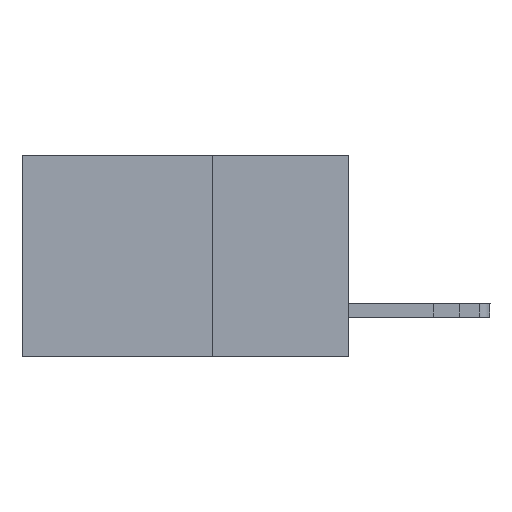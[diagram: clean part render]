
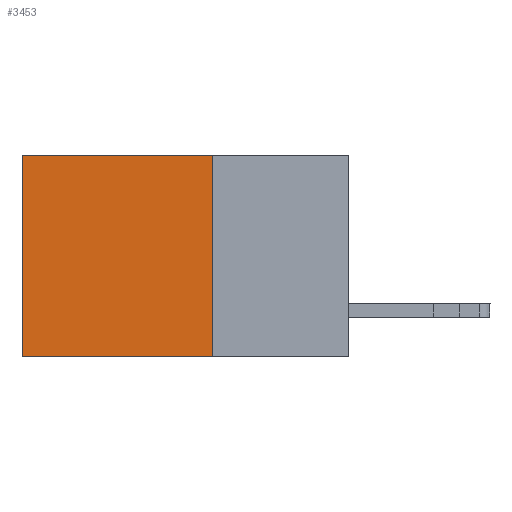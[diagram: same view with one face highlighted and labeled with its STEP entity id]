
A CAD part, left-side view. The second image highlights one B-rep face of the part: STEP entity #3453.
In plain terms, the highlighted planar face has unit normal (-1, 0, 0).
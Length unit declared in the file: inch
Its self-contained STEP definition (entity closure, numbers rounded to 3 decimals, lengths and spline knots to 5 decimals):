
#964 = EDGE_CURVE ( 'NONE', #2668, #8851, #7238, .T. ) ;
#1015 = VECTOR ( 'NONE', #5748, 39.37008 ) ;
#1141 = CARTESIAN_POINT ( 'NONE',  ( 0.2615, 0.25, -0.37 ) ) ;
#1607 = LINE ( 'NONE', #3396, #9876 ) ;
#2038 = ORIENTED_EDGE ( 'NONE', *, *, #2424, .T. ) ;
#2151 = EDGE_CURVE ( 'NONE', #8851, #8333, #9341, .T. ) ;
#2341 = VERTEX_POINT ( 'NONE', #6383 ) ;
#2424 = EDGE_CURVE ( 'NONE', #2341, #8333, #9096, .T. ) ;
#2668 = VERTEX_POINT ( 'NONE', #3450 ) ;
#3125 = CARTESIAN_POINT ( 'NONE',  ( 0.2615, 0.25, -0.37 ) ) ;
#3248 = DIRECTION ( 'NONE',  ( 1., 0., 0. ) ) ;
#3284 = ORIENTED_EDGE ( 'NONE', *, *, #964, .F. ) ;
#3394 = VECTOR ( 'NONE', #6154, 39.37008 ) ;
#3396 = CARTESIAN_POINT ( 'NONE',  ( 0.2615, 0.25, 0. ) ) ;
#3450 = CARTESIAN_POINT ( 'NONE',  ( 0.2615, 0.25, 0. ) ) ;
#3453 = ADVANCED_FACE ( 'NONE', ( #11069 ), #10953, .F. ) ;
#3691 = EDGE_LOOP ( 'NONE', ( #2038, #5151, #3284, #9716 ) ) ;
#4535 = VECTOR ( 'NONE', #10813, 39.37008 ) ;
#5151 = ORIENTED_EDGE ( 'NONE', *, *, #2151, .F. ) ;
#5748 = DIRECTION ( 'NONE',  ( 0., 1., 0. ) ) ;
#5921 = CARTESIAN_POINT ( 'NONE',  ( 0.2615, 0.25, -0.37 ) ) ;
#6154 = DIRECTION ( 'NONE',  ( 0., 0., -1. ) ) ;
#6383 = CARTESIAN_POINT ( 'NONE',  ( 0.2615, 0.6, 0. ) ) ;
#6750 = DIRECTION ( 'NONE',  ( 0., 0., -1. ) ) ;
#7238 = LINE ( 'NONE', #1141, #3394 ) ;
#7282 = EDGE_CURVE ( 'NONE', #2668, #2341, #1607, .T. ) ;
#7301 = CARTESIAN_POINT ( 'NONE',  ( 0.2615, 0.6, -0.37 ) ) ;
#7349 = AXIS2_PLACEMENT_3D ( 'NONE', #3125, #3248, #6750 ) ;
#7429 = CARTESIAN_POINT ( 'NONE',  ( 0.2615, 0.6, -0.37 ) ) ;
#7810 = CARTESIAN_POINT ( 'NONE',  ( 0.2615, 0.25, -0.37 ) ) ;
#8333 = VERTEX_POINT ( 'NONE', #7429 ) ;
#8693 = DIRECTION ( 'NONE',  ( 0., 1., 0. ) ) ;
#8851 = VERTEX_POINT ( 'NONE', #7810 ) ;
#9096 = LINE ( 'NONE', #7301, #4535 ) ;
#9341 = LINE ( 'NONE', #5921, #1015 ) ;
#9716 = ORIENTED_EDGE ( 'NONE', *, *, #7282, .T. ) ;
#9876 = VECTOR ( 'NONE', #8693, 39.37008 ) ;
#10813 = DIRECTION ( 'NONE',  ( 0., 0., -1. ) ) ;
#10953 = PLANE ( 'NONE',  #7349 ) ;
#11069 = FACE_OUTER_BOUND ( 'NONE', #3691, .T. ) ;
